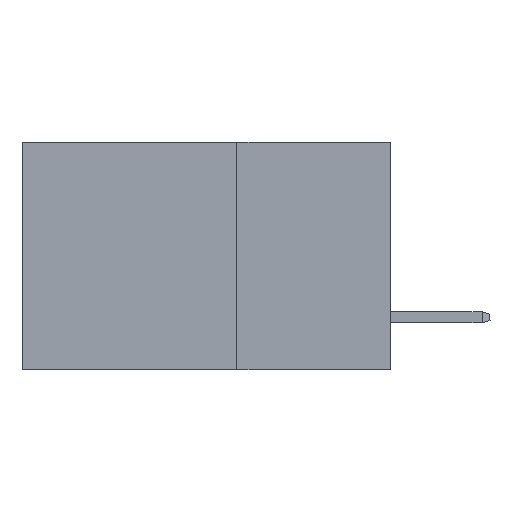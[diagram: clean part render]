
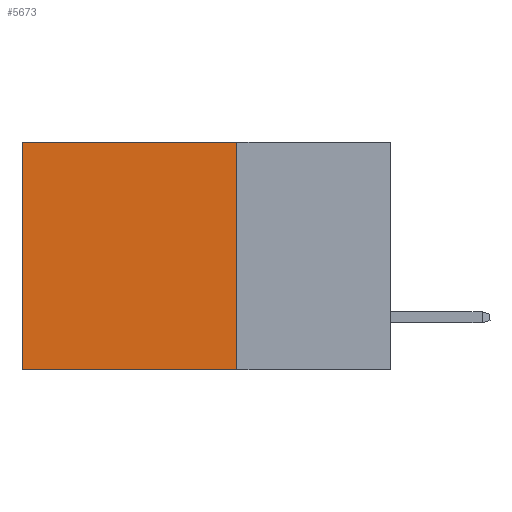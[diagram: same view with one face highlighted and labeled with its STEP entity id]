
A CAD part, left-side view. The second image highlights one B-rep face of the part: STEP entity #5673.
In plain terms, the highlighted planar face has unit normal (-1, 0, 0).
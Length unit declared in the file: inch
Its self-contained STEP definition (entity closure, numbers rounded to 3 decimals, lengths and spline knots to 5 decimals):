
#738 = VECTOR ( 'NONE', #4288, 39.37008 ) ;
#909 = LINE ( 'NONE', #6867, #8175 ) ;
#1563 = VERTEX_POINT ( 'NONE', #5964 ) ;
#1788 = CARTESIAN_POINT ( 'NONE',  ( 0.2875, 0.25, 0. ) ) ;
#2430 = LINE ( 'NONE', #12163, #4335 ) ;
#2887 = EDGE_CURVE ( 'NONE', #6496, #1563, #10938, .T. ) ;
#3340 = ORIENTED_EDGE ( 'NONE', *, *, #2887, .F. ) ;
#3802 = AXIS2_PLACEMENT_3D ( 'NONE', #1788, #5581, #12241 ) ;
#4203 = CARTESIAN_POINT ( 'NONE',  ( 0.2875, 0.6, 0. ) ) ;
#4288 = DIRECTION ( 'NONE',  ( 0., 1., 0. ) ) ;
#4335 = VECTOR ( 'NONE', #5509, 39.37008 ) ;
#4844 = DIRECTION ( 'NONE',  ( 0., 0., -1. ) ) ;
#5104 = ORIENTED_EDGE ( 'NONE', *, *, #10987, .F. ) ;
#5509 = DIRECTION ( 'NONE',  ( 0., 0., -1. ) ) ;
#5581 = DIRECTION ( 'NONE',  ( 1., 0., 0. ) ) ;
#5629 = EDGE_CURVE ( 'NONE', #10908, #11093, #2430, .T. ) ;
#5673 = ADVANCED_FACE ( 'NONE', ( #11045 ), #11298, .F. ) ;
#5745 = LINE ( 'NONE', #6197, #738 ) ;
#5964 = CARTESIAN_POINT ( 'NONE',  ( 0.2875, 0.25, -0.37 ) ) ;
#6197 = CARTESIAN_POINT ( 'NONE',  ( 0.2875, 0.25, -0.37 ) ) ;
#6496 = VERTEX_POINT ( 'NONE', #11473 ) ;
#6749 = CARTESIAN_POINT ( 'NONE',  ( 0.2875, 0.25, 0. ) ) ;
#6867 = CARTESIAN_POINT ( 'NONE',  ( 0.2875, 0.25, 0. ) ) ;
#7121 = EDGE_CURVE ( 'NONE', #6496, #10908, #909, .T. ) ;
#8175 = VECTOR ( 'NONE', #10710, 39.37008 ) ;
#9389 = ORIENTED_EDGE ( 'NONE', *, *, #7121, .T. ) ;
#9662 = ORIENTED_EDGE ( 'NONE', *, *, #5629, .T. ) ;
#10626 = VECTOR ( 'NONE', #4844, 39.37008 ) ;
#10710 = DIRECTION ( 'NONE',  ( 0., 1., 0. ) ) ;
#10908 = VERTEX_POINT ( 'NONE', #4203 ) ;
#10938 = LINE ( 'NONE', #6749, #10626 ) ;
#10987 = EDGE_CURVE ( 'NONE', #1563, #11093, #5745, .T. ) ;
#11045 = FACE_OUTER_BOUND ( 'NONE', #11503, .T. ) ;
#11093 = VERTEX_POINT ( 'NONE', #12065 ) ;
#11298 = PLANE ( 'NONE',  #3802 ) ;
#11473 = CARTESIAN_POINT ( 'NONE',  ( 0.2875, 0.25, 0. ) ) ;
#11503 = EDGE_LOOP ( 'NONE', ( #9662, #5104, #3340, #9389 ) ) ;
#12065 = CARTESIAN_POINT ( 'NONE',  ( 0.2875, 0.6, -0.37 ) ) ;
#12163 = CARTESIAN_POINT ( 'NONE',  ( 0.2875, 0.6, 0. ) ) ;
#12241 = DIRECTION ( 'NONE',  ( 0., 0., -1. ) ) ;
